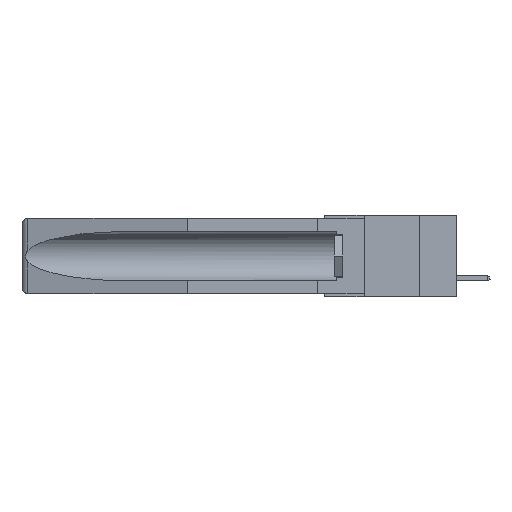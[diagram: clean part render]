
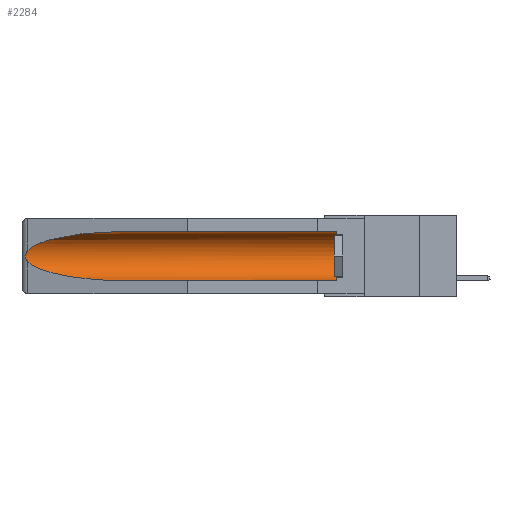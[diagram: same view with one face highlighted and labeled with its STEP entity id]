
A CAD part, left-side view. The second image highlights one B-rep face of the part: STEP entity #2284.
In plain terms, the highlighted cylindrical face has radius 2.857 mm (diameter 5.715 mm), a partial arc.
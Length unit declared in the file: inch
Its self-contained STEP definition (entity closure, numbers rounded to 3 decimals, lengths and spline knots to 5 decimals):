
#156 = CARTESIAN_POINT ( 'NONE',  ( 0.25451, 1.48313, -0.24835 ) ) ;
#585 = CARTESIAN_POINT ( 'NONE',  ( 0.155, -0.30754, -0.1715 ) ) ;
#831 = CARTESIAN_POINT ( 'NONE',  ( 0.26537, 1.52718, -0.14972 ) ) ;
#865 = CARTESIAN_POINT ( 'NONE',  ( 0.26537, 1.52718, -0.14972 ) ) ;
#1496 = VECTOR ( 'NONE', #13320, 39.37008 ) ;
#1831 = CARTESIAN_POINT ( 'NONE',  ( 0.155, 1.07973, -0.284 ) ) ;
#1940 = EDGE_CURVE ( 'NONE', #16723, #8307, #16234, .T. ) ;
#2284 = ADVANCED_FACE ( 'NONE', ( #11445 ), #7147, .F. ) ;
#2473 = DIRECTION ( 'NONE',  ( 0., 1., 0. ) ) ;
#2965 = CARTESIAN_POINT ( 'NONE',  ( 0.26537, 1.52718, -0.14972 ) ) ;
#3038 = CARTESIAN_POINT ( 'NONE',  ( 0.26597, 1.52961, -0.15275 ) ) ;
#3402 = CARTESIAN_POINT ( 'NONE',  ( 0.21114, 1.30732, -0.284 ) ) ;
#3873 = AXIS2_PLACEMENT_3D ( 'NONE', #20886, #6459, #12885 ) ;
#3945 = VECTOR ( 'NONE', #4562, 39.37008 ) ;
#4129 = DIRECTION ( 'NONE',  ( 0., 0., 1. ) ) ;
#4562 = DIRECTION ( 'NONE',  ( 0., 1., 0. ) ) ;
#4985 = ORIENTED_EDGE ( 'NONE', *, *, #1940, .T. ) ;
#5523 = VERTEX_POINT ( 'NONE', #7523 ) ;
#5666 = VERTEX_POINT ( 'NONE', #11367 ) ;
#5718 = EDGE_CURVE ( 'NONE', #11604, #16575, #11928, .T. ) ;
#6064 = CARTESIAN_POINT ( 'NONE',  ( 0.26597, 1.5296, -0.19026 ) ) ;
#6229 = CARTESIAN_POINT ( 'NONE',  ( 0.155, -0.30754, -0.059 ) ) ;
#6267 = CARTESIAN_POINT ( 'NONE',  ( 0.26654, 1.53092, -0.15636 ) ) ;
#6338 = EDGE_CURVE ( 'NONE', #5523, #16575, #10538, .T. ) ;
#6459 = DIRECTION ( 'NONE',  ( 0., -1., 0. ) ) ;
#7147 = CYLINDRICAL_SURFACE ( 'NONE', #13696, 0.1125 ) ;
#7523 = CARTESIAN_POINT ( 'NONE',  ( 0.155, 0.126, -0.284 ) ) ;
#7710 = CARTESIAN_POINT ( 'NONE',  ( 0.26537, 1.52718, -0.19328 ) ) ;
#7777 = CARTESIAN_POINT ( 'NONE',  ( 0.2675, 1.53308, -0.17534 ) ) ;
#8307 = VERTEX_POINT ( 'NONE', #831 ) ;
#8538 = CARTESIAN_POINT ( 'NONE',  ( 0.155, 1.07973, -0.059 ) ) ;
#8966 = EDGE_CURVE ( 'NONE', #5666, #16723, #17326, .T. ) ;
#9023 = EDGE_LOOP ( 'NONE', ( #4985, #14822, #20242, #15759, #11434, #13450 ) ) ;
#9071 = CARTESIAN_POINT ( 'NONE',  ( 0.25451, 1.48313, -0.09465 ) ) ;
#9214 = CARTESIAN_POINT ( 'NONE',  ( 0.21114, 1.30732, -0.059 ) ) ;
#9537 = CARTESIAN_POINT ( 'NONE',  ( 0.2673, 1.5327, -0.16383 ) ) ;
#10538 = LINE ( 'NONE', #16163, #1496 ) ;
#11367 = CARTESIAN_POINT ( 'NONE',  ( 0.155, 0.126, -0.059 ) ) ;
#11434 = ORIENTED_EDGE ( 'NONE', *, *, #17628, .T. ) ;
#11445 = FACE_OUTER_BOUND ( 'NONE', #9023, .T. ) ;
#11604 = VERTEX_POINT ( 'NONE', #12493 ) ;
#11928 =( BOUNDED_CURVE ( )  B_SPLINE_CURVE ( 3, ( #12908, #156, #3402, #16327 ),
 .UNSPECIFIED., .F., .F. ) 
 B_SPLINE_CURVE_WITH_KNOTS ( ( 4, 4 ),
 ( 0.1948, 1.5708 ),
 .UNSPECIFIED. ) 
 CURVE ( )  GEOMETRIC_REPRESENTATION_ITEM ( )  RATIONAL_B_SPLINE_CURVE ( ( 1., 0.848, 0.848, 1. ) ) 
 REPRESENTATION_ITEM ( '' )  );
#12493 = CARTESIAN_POINT ( 'NONE',  ( 0.26537, 1.52718, -0.19328 ) ) ;
#12885 = DIRECTION ( 'NONE',  ( 0., 0., 1. ) ) ;
#12908 = CARTESIAN_POINT ( 'NONE',  ( 0.26537, 1.52718, -0.19328 ) ) ;
#13320 = DIRECTION ( 'NONE',  ( 0., 1., 0. ) ) ;
#13450 = ORIENTED_EDGE ( 'NONE', *, *, #8966, .T. ) ;
#13696 = AXIS2_PLACEMENT_3D ( 'NONE', #585, #2473, #4129 ) ;
#13934 = CARTESIAN_POINT ( 'NONE',  ( 0.155, 1.07973, -0.059 ) ) ;
#14194 = CARTESIAN_POINT ( 'NONE',  ( 0.2673, 1.53269, -0.17917 ) ) ;
#14822 = ORIENTED_EDGE ( 'NONE', *, *, #18801, .T. ) ;
#15759 = ORIENTED_EDGE ( 'NONE', *, *, #6338, .F. ) ;
#16163 = CARTESIAN_POINT ( 'NONE',  ( 0.155, -0.30754, -0.284 ) ) ;
#16234 =( BOUNDED_CURVE ( )  B_SPLINE_CURVE ( 3, ( #13934, #9214, #9071, #865 ),
 .UNSPECIFIED., .F., .F. ) 
 B_SPLINE_CURVE_WITH_KNOTS ( ( 4, 4 ),
 ( 4.71239, 6.08839 ),
 .UNSPECIFIED. ) 
 CURVE ( )  GEOMETRIC_REPRESENTATION_ITEM ( )  RATIONAL_B_SPLINE_CURVE ( ( 1., 0.848, 0.848, 1. ) ) 
 REPRESENTATION_ITEM ( '' )  );
#16327 = CARTESIAN_POINT ( 'NONE',  ( 0.155, 1.07973, -0.284 ) ) ;
#16575 = VERTEX_POINT ( 'NONE', #1831 ) ;
#16623 = B_SPLINE_CURVE_WITH_KNOTS ( 'NONE', 3,
 ( #2965, #3038, #6267, #9537, #19584, #7777, #14194, #20840, #6064, #7710 ),
 .UNSPECIFIED., .F., .F.,
 ( 4, 2, 2, 2, 4 ),
 ( 0., 0.00029, 0.00058, 0.00087, 0.00117 ),
 .UNSPECIFIED. ) ;
#16723 = VERTEX_POINT ( 'NONE', #8538 ) ;
#17326 = LINE ( 'NONE', #6229, #3945 ) ;
#17628 = EDGE_CURVE ( 'NONE', #5523, #5666, #19389, .T. ) ;
#18801 = EDGE_CURVE ( 'NONE', #8307, #11604, #16623, .T. ) ;
#19389 = CIRCLE ( 'NONE', #3873, 0.1125 ) ;
#19584 = CARTESIAN_POINT ( 'NONE',  ( 0.2675, 1.53308, -0.16763 ) ) ;
#20242 = ORIENTED_EDGE ( 'NONE', *, *, #5718, .T. ) ;
#20840 = CARTESIAN_POINT ( 'NONE',  ( 0.26655, 1.53094, -0.18657 ) ) ;
#20886 = CARTESIAN_POINT ( 'NONE',  ( 0.155, 0.126, -0.1715 ) ) ;
